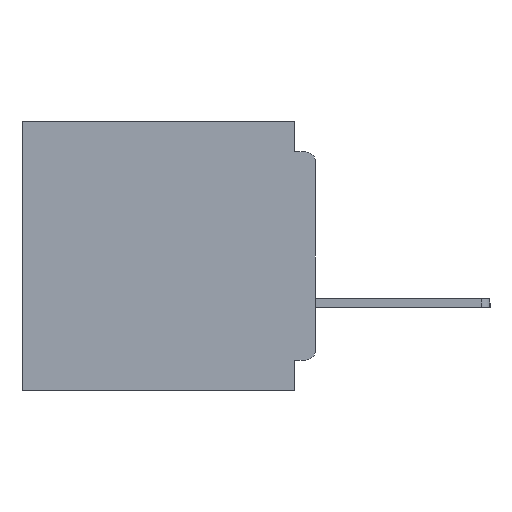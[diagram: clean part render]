
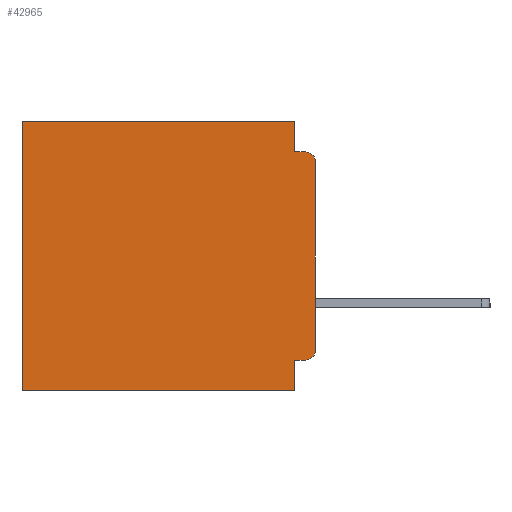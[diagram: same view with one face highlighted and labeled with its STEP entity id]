
A CAD part, left-side view. The second image highlights one B-rep face of the part: STEP entity #42965.
In plain terms, the highlighted planar face has unit normal (-1, 0, 0).
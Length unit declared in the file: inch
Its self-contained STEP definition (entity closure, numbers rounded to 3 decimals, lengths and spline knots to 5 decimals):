
#63 = ORIENTED_EDGE ( 'NONE', *, *, #15892, .F. ) ;
#926 = VERTEX_POINT ( 'NONE', #13859 ) ;
#1842 = ORIENTED_EDGE ( 'NONE', *, *, #35102, .T. ) ;
#2480 = LINE ( 'NONE', #30730, #40144 ) ;
#2866 = CARTESIAN_POINT ( 'NONE',  ( 0.3, 0.031, -0.4 ) ) ;
#3447 = VECTOR ( 'NONE', #20222, 39.37008 ) ;
#4273 = PLANE ( 'NONE',  #32499 ) ;
#4510 = DIRECTION ( 'NONE',  ( 0., 0., -1. ) ) ;
#5098 = DIRECTION ( 'NONE',  ( 0., 0., -1. ) ) ;
#5578 = CARTESIAN_POINT ( 'NONE',  ( 0.3, 0.015, -0.045 ) ) ;
#5633 = ORIENTED_EDGE ( 'NONE', *, *, #10304, .T. ) ;
#5913 = ORIENTED_EDGE ( 'NONE', *, *, #13694, .F. ) ;
#6213 = CARTESIAN_POINT ( 'NONE',  ( 0.3, 0.031, -0.355 ) ) ;
#6505 = VECTOR ( 'NONE', #19395, 39.37008 ) ;
#7045 = AXIS2_PLACEMENT_3D ( 'NONE', #15483, #40834, #19135 ) ;
#7097 = ORIENTED_EDGE ( 'NONE', *, *, #13523, .T. ) ;
#8543 = VERTEX_POINT ( 'NONE', #23269 ) ;
#9375 = LINE ( 'NONE', #18809, #27622 ) ;
#9517 = EDGE_LOOP ( 'NONE', ( #38399, #1842, #42852, #28224, #7097, #18600, #5913, #30137, #63, #5633 ) ) ;
#10275 = CIRCLE ( 'NONE', #7045, 0.015 ) ;
#10300 = DIRECTION ( 'NONE',  ( 0., 0., -1. ) ) ;
#10304 = EDGE_CURVE ( 'NONE', #39593, #42067, #10275, .T. ) ;
#10561 = LINE ( 'NONE', #20968, #46792 ) ;
#12397 = VERTEX_POINT ( 'NONE', #42633 ) ;
#13523 = EDGE_CURVE ( 'NONE', #30186, #12397, #16358, .T. ) ;
#13564 = CIRCLE ( 'NONE', #44865, 0.015 ) ;
#13694 = EDGE_CURVE ( 'NONE', #43549, #926, #10561, .T. ) ;
#13859 = CARTESIAN_POINT ( 'NONE',  ( 0.3, 0.437, -0.4 ) ) ;
#14267 = DIRECTION ( 'NONE',  ( -1., 0., 0. ) ) ;
#14439 = LINE ( 'NONE', #41858, #3447 ) ;
#15440 = CARTESIAN_POINT ( 'NONE',  ( 0.3, 0., -0.4 ) ) ;
#15483 = CARTESIAN_POINT ( 'NONE',  ( 0.3, 0.015, -0.34 ) ) ;
#15737 = CARTESIAN_POINT ( 'NONE',  ( 0.3, 0., 0. ) ) ;
#15892 = EDGE_CURVE ( 'NONE', #39593, #22567, #45497, .T. ) ;
#16105 = CARTESIAN_POINT ( 'NONE',  ( 0.3, 0.015, -0.355 ) ) ;
#16358 = LINE ( 'NONE', #15737, #6505 ) ;
#18600 = ORIENTED_EDGE ( 'NONE', *, *, #39599, .T. ) ;
#18809 = CARTESIAN_POINT ( 'NONE',  ( 0.3, 0.031, 0. ) ) ;
#19101 = DIRECTION ( 'NONE',  ( 0., 0., -1. ) ) ;
#19135 = DIRECTION ( 'NONE',  ( 0., 0., -1. ) ) ;
#19310 = EDGE_CURVE ( 'NONE', #22567, #43549, #42752, .T. ) ;
#19395 = DIRECTION ( 'NONE',  ( 0., 1., 0. ) ) ;
#20222 = DIRECTION ( 'NONE',  ( 0., -1., 0. ) ) ;
#20476 = VERTEX_POINT ( 'NONE', #46006 ) ;
#20968 = CARTESIAN_POINT ( 'NONE',  ( 0.3, 0., -0.4 ) ) ;
#20978 = FACE_OUTER_BOUND ( 'NONE', #9517, .T. ) ;
#21667 = VECTOR ( 'NONE', #4510, 39.37008 ) ;
#22455 = VERTEX_POINT ( 'NONE', #5578 ) ;
#22458 = DIRECTION ( 'NONE',  ( 0., 0., -1. ) ) ;
#22567 = VERTEX_POINT ( 'NONE', #6213 ) ;
#22828 = CARTESIAN_POINT ( 'NONE',  ( 0.3, 0., -0.4 ) ) ;
#23269 = CARTESIAN_POINT ( 'NONE',  ( 0.3, 0., -0.06 ) ) ;
#24623 = DIRECTION ( 'NONE',  ( 0., 1., 0. ) ) ;
#27622 = VECTOR ( 'NONE', #22458, 39.37008 ) ;
#28224 = ORIENTED_EDGE ( 'NONE', *, *, #29364, .F. ) ;
#29364 = EDGE_CURVE ( 'NONE', #30186, #20476, #9375, .T. ) ;
#30137 = ORIENTED_EDGE ( 'NONE', *, *, #19310, .F. ) ;
#30186 = VERTEX_POINT ( 'NONE', #37772 ) ;
#30730 = CARTESIAN_POINT ( 'NONE',  ( 0.3, 0.437, -0.4 ) ) ;
#31336 = LINE ( 'NONE', #22828, #21667 ) ;
#32039 = CARTESIAN_POINT ( 'NONE',  ( 0.3, 0., -0.34 ) ) ;
#32499 = AXIS2_PLACEMENT_3D ( 'NONE', #15440, #40793, #19101 ) ;
#33210 = VECTOR ( 'NONE', #10300, 39.37008 ) ;
#34123 = EDGE_CURVE ( 'NONE', #8543, #42067, #31336, .T. ) ;
#35102 = EDGE_CURVE ( 'NONE', #8543, #22455, #13564, .T. ) ;
#35997 = VECTOR ( 'NONE', #37287, 39.37008 ) ;
#36054 = CARTESIAN_POINT ( 'NONE',  ( 0.3, 0.015, -0.06 ) ) ;
#36984 = CARTESIAN_POINT ( 'NONE',  ( 0.3, 0.031, -0.4 ) ) ;
#37287 = DIRECTION ( 'NONE',  ( 0., 1., 0. ) ) ;
#37772 = CARTESIAN_POINT ( 'NONE',  ( 0.3, 0.031, 0. ) ) ;
#38399 = ORIENTED_EDGE ( 'NONE', *, *, #34123, .F. ) ;
#39593 = VERTEX_POINT ( 'NONE', #16105 ) ;
#39599 = EDGE_CURVE ( 'NONE', #12397, #926, #2480, .T. ) ;
#39642 = DIRECTION ( 'NONE',  ( 0., 0., -1. ) ) ;
#40144 = VECTOR ( 'NONE', #5098, 39.37008 ) ;
#40580 = CARTESIAN_POINT ( 'NONE',  ( 0.3, 0., -0.355 ) ) ;
#40793 = DIRECTION ( 'NONE',  ( 1., 0., 0. ) ) ;
#40834 = DIRECTION ( 'NONE',  ( -1., 0., 0. ) ) ;
#41858 = CARTESIAN_POINT ( 'NONE',  ( 0.3, 0., -0.045 ) ) ;
#42067 = VERTEX_POINT ( 'NONE', #32039 ) ;
#42633 = CARTESIAN_POINT ( 'NONE',  ( 0.3, 0.437, 0. ) ) ;
#42752 = LINE ( 'NONE', #2866, #33210 ) ;
#42852 = ORIENTED_EDGE ( 'NONE', *, *, #45503, .F. ) ;
#42965 = ADVANCED_FACE ( 'NONE', ( #20978 ), #4273, .F. ) ;
#43549 = VERTEX_POINT ( 'NONE', #36984 ) ;
#44865 = AXIS2_PLACEMENT_3D ( 'NONE', #36054, #14267, #39642 ) ;
#45497 = LINE ( 'NONE', #40580, #35997 ) ;
#45503 = EDGE_CURVE ( 'NONE', #20476, #22455, #14439, .T. ) ;
#46006 = CARTESIAN_POINT ( 'NONE',  ( 0.3, 0.031, -0.045 ) ) ;
#46792 = VECTOR ( 'NONE', #24623, 39.37008 ) ;
